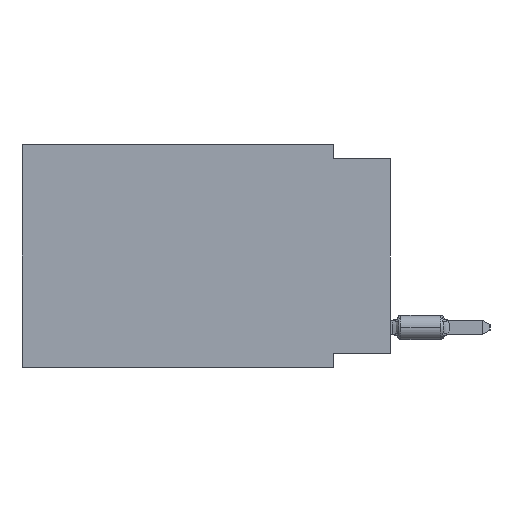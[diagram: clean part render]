
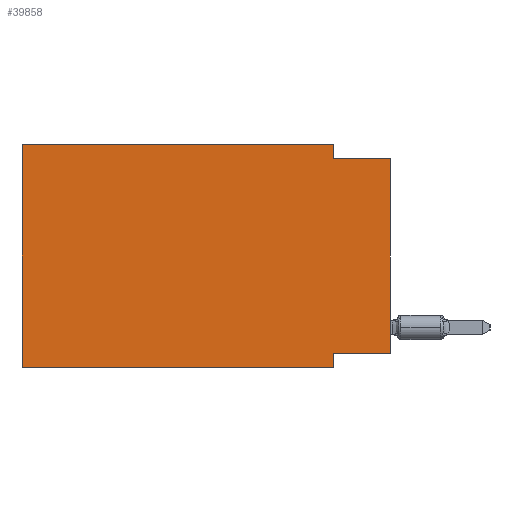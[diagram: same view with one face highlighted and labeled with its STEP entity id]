
A CAD part, left-side view. The second image highlights one B-rep face of the part: STEP entity #39858.
In plain terms, the highlighted planar face has unit normal (-1, 0, 0).
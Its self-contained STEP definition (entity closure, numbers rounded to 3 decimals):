
#849 = CARTESIAN_POINT ( 'NONE',  ( 0., 0., -9.271 ) ) ;
#2263 = DIRECTION ( 'NONE',  ( 0., -1., 0. ) ) ;
#3723 = CARTESIAN_POINT ( 'NONE',  ( 0., 16.383, 0. ) ) ;
#3745 = ORIENTED_EDGE ( 'NONE', *, *, #18832, .F. ) ;
#4031 = VERTEX_POINT ( 'NONE', #11174 ) ;
#6038 = VECTOR ( 'NONE', #53087, 1000. ) ;
#6187 = CARTESIAN_POINT ( 'NONE',  ( 0., 16.383, -9.906 ) ) ;
#6497 = VERTEX_POINT ( 'NONE', #57957 ) ;
#7420 = VECTOR ( 'NONE', #40704, 1000. ) ;
#8522 = CARTESIAN_POINT ( 'NONE',  ( 0., 2.54, -0.635 ) ) ;
#9595 = ORIENTED_EDGE ( 'NONE', *, *, #54116, .F. ) ;
#9653 = VERTEX_POINT ( 'NONE', #15706 ) ;
#10108 = VERTEX_POINT ( 'NONE', #849 ) ;
#11174 = CARTESIAN_POINT ( 'NONE',  ( 0., 2.54, -9.906 ) ) ;
#11215 = VECTOR ( 'NONE', #33473, 1000. ) ;
#12297 = LINE ( 'NONE', #48046, #24995 ) ;
#14554 = EDGE_CURVE ( 'NONE', #51169, #23781, #22195, .T. ) ;
#15442 = EDGE_CURVE ( 'NONE', #10108, #9653, #22620, .T. ) ;
#15706 = CARTESIAN_POINT ( 'NONE',  ( 0., 0., -0.635 ) ) ;
#16465 = DIRECTION ( 'NONE',  ( 1., 0., 0. ) ) ;
#17245 = VECTOR ( 'NONE', #57950, 1000. ) ;
#17321 = CARTESIAN_POINT ( 'NONE',  ( 0., 16.383, 0. ) ) ;
#17530 = VECTOR ( 'NONE', #2263, 1000. ) ;
#17873 = ORIENTED_EDGE ( 'NONE', *, *, #18244, .F. ) ;
#18244 = EDGE_CURVE ( 'NONE', #47287, #29417, #54400, .T. ) ;
#18832 = EDGE_CURVE ( 'NONE', #6497, #4031, #50568, .T. ) ;
#18927 = DIRECTION ( 'NONE',  ( 0., 0., -1. ) ) ;
#19130 = ORIENTED_EDGE ( 'NONE', *, *, #19833, .F. ) ;
#19603 = EDGE_LOOP ( 'NONE', ( #23153, #20265, #17873, #9595, #49685, #47242, #3745, #19130 ) ) ;
#19833 = EDGE_CURVE ( 'NONE', #10108, #6497, #12297, .T. ) ;
#20265 = ORIENTED_EDGE ( 'NONE', *, *, #42398, .F. ) ;
#20289 = CARTESIAN_POINT ( 'NONE',  ( 0., 16.383, 0. ) ) ;
#20540 = EDGE_CURVE ( 'NONE', #51169, #4031, #25122, .T. ) ;
#21366 = DIRECTION ( 'NONE',  ( 0., 1., 0. ) ) ;
#22195 = LINE ( 'NONE', #3723, #17245 ) ;
#22620 = LINE ( 'NONE', #45177, #6038 ) ;
#22826 = CARTESIAN_POINT ( 'NONE',  ( 0., 0., -0.635 ) ) ;
#23153 = ORIENTED_EDGE ( 'NONE', *, *, #15442, .T. ) ;
#23781 = VERTEX_POINT ( 'NONE', #46672 ) ;
#24192 = CARTESIAN_POINT ( 'NONE',  ( 0., 2.54, 0. ) ) ;
#24934 = AXIS2_PLACEMENT_3D ( 'NONE', #17321, #16465, #53073 ) ;
#24995 = VECTOR ( 'NONE', #21366, 1000. ) ;
#25122 = LINE ( 'NONE', #25699, #17530 ) ;
#25699 = CARTESIAN_POINT ( 'NONE',  ( 0., 16.383, -9.906 ) ) ;
#26901 = CARTESIAN_POINT ( 'NONE',  ( 0., 2.54, 0. ) ) ;
#29417 = VERTEX_POINT ( 'NONE', #8522 ) ;
#33473 = DIRECTION ( 'NONE',  ( 0., -1., 0. ) ) ;
#34909 = PLANE ( 'NONE',  #24934 ) ;
#39858 = ADVANCED_FACE ( 'NONE', ( #57483 ), #34909, .F. ) ;
#40704 = DIRECTION ( 'NONE',  ( 0., -1., 0. ) ) ;
#42398 = EDGE_CURVE ( 'NONE', #29417, #9653, #45091, .T. ) ;
#45091 = LINE ( 'NONE', #22826, #7420 ) ;
#45177 = CARTESIAN_POINT ( 'NONE',  ( 0., 0., 0. ) ) ;
#45893 = DIRECTION ( 'NONE',  ( 0., 0., -1. ) ) ;
#46672 = CARTESIAN_POINT ( 'NONE',  ( 0., 16.383, 0. ) ) ;
#47242 = ORIENTED_EDGE ( 'NONE', *, *, #20540, .T. ) ;
#47287 = VERTEX_POINT ( 'NONE', #26901 ) ;
#48046 = CARTESIAN_POINT ( 'NONE',  ( 0., 0., -9.271 ) ) ;
#49391 = VECTOR ( 'NONE', #45893, 1000. ) ;
#49685 = ORIENTED_EDGE ( 'NONE', *, *, #14554, .F. ) ;
#50280 = CARTESIAN_POINT ( 'NONE',  ( 0., 2.54, -9.906 ) ) ;
#50301 = VECTOR ( 'NONE', #18927, 1000. ) ;
#50568 = LINE ( 'NONE', #50280, #49391 ) ;
#51078 = LINE ( 'NONE', #20289, #11215 ) ;
#51169 = VERTEX_POINT ( 'NONE', #6187 ) ;
#53073 = DIRECTION ( 'NONE',  ( 0., 0., -1. ) ) ;
#53087 = DIRECTION ( 'NONE',  ( 0., 0., 1. ) ) ;
#54116 = EDGE_CURVE ( 'NONE', #23781, #47287, #51078, .T. ) ;
#54400 = LINE ( 'NONE', #24192, #50301 ) ;
#57483 = FACE_OUTER_BOUND ( 'NONE', #19603, .T. ) ;
#57950 = DIRECTION ( 'NONE',  ( 0., 0., 1. ) ) ;
#57957 = CARTESIAN_POINT ( 'NONE',  ( 0., 2.54, -9.271 ) ) ;
